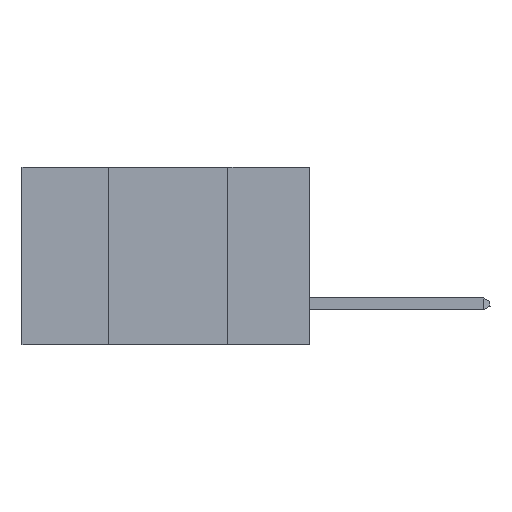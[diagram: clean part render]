
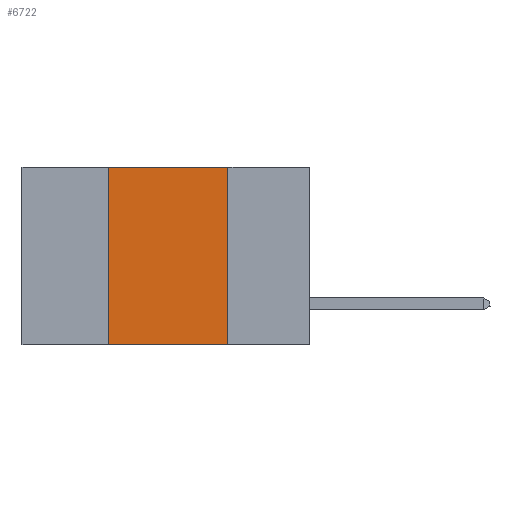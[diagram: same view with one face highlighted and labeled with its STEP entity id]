
A CAD part, left-side view. The second image highlights one B-rep face of the part: STEP entity #6722.
In plain terms, the highlighted planar face has unit normal (-1, 0, 0).
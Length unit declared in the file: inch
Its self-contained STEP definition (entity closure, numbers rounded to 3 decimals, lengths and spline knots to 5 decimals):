
#813 = LINE ( 'NONE', #24968, #1257 ) ;
#1054 = EDGE_CURVE ( 'NONE', #26137, #22305, #813, .T. ) ;
#1257 = VECTOR ( 'NONE', #18812, 39.37008 ) ;
#2636 = VERTEX_POINT ( 'NONE', #23611 ) ;
#5283 = LINE ( 'NONE', #9073, #12096 ) ;
#5435 = ORIENTED_EDGE ( 'NONE', *, *, #1054, .F. ) ;
#6722 = ADVANCED_FACE ( 'NONE', ( #33055 ), #16231, .F. ) ;
#7300 = CARTESIAN_POINT ( 'NONE',  ( 0., 0.6, 0. ) ) ;
#7421 = LINE ( 'NONE', #27315, #16544 ) ;
#9073 = CARTESIAN_POINT ( 'NONE',  ( 0., 0.42, 0. ) ) ;
#9664 = LINE ( 'NONE', #26863, #32115 ) ;
#11010 = EDGE_CURVE ( 'NONE', #23746, #26137, #7421, .T. ) ;
#12092 = EDGE_CURVE ( 'NONE', #2636, #22305, #9664, .T. ) ;
#12096 = VECTOR ( 'NONE', #26700, 39.37008 ) ;
#12722 = EDGE_LOOP ( 'NONE', ( #5435, #26218, #24633, #35678 ) ) ;
#13685 = DIRECTION ( 'NONE',  ( 0., 0., -1. ) ) ;
#14954 = DIRECTION ( 'NONE',  ( 0., -1., 0. ) ) ;
#15015 = AXIS2_PLACEMENT_3D ( 'NONE', #7300, #28284, #13685 ) ;
#16045 = DIRECTION ( 'NONE',  ( 0., -1., 0. ) ) ;
#16231 = PLANE ( 'NONE',  #15015 ) ;
#16544 = VECTOR ( 'NONE', #16045, 39.37008 ) ;
#18674 = CARTESIAN_POINT ( 'NONE',  ( 0., 0.17, -0.37 ) ) ;
#18812 = DIRECTION ( 'NONE',  ( 0., 0., -1. ) ) ;
#20277 = CARTESIAN_POINT ( 'NONE',  ( 0., 0.17, 0. ) ) ;
#21749 = CARTESIAN_POINT ( 'NONE',  ( 0., 0.42, 0. ) ) ;
#22305 = VERTEX_POINT ( 'NONE', #18674 ) ;
#23611 = CARTESIAN_POINT ( 'NONE',  ( 0., 0.42, -0.37 ) ) ;
#23746 = VERTEX_POINT ( 'NONE', #21749 ) ;
#24633 = ORIENTED_EDGE ( 'NONE', *, *, #24878, .F. ) ;
#24878 = EDGE_CURVE ( 'NONE', #2636, #23746, #5283, .T. ) ;
#24968 = CARTESIAN_POINT ( 'NONE',  ( 0., 0.17, 0. ) ) ;
#26137 = VERTEX_POINT ( 'NONE', #20277 ) ;
#26218 = ORIENTED_EDGE ( 'NONE', *, *, #11010, .F. ) ;
#26700 = DIRECTION ( 'NONE',  ( 0., 0., 1. ) ) ;
#26863 = CARTESIAN_POINT ( 'NONE',  ( 0., 0.6, -0.37 ) ) ;
#27315 = CARTESIAN_POINT ( 'NONE',  ( 0., 0.6, 0. ) ) ;
#28284 = DIRECTION ( 'NONE',  ( 1., 0., 0. ) ) ;
#32115 = VECTOR ( 'NONE', #14954, 39.37008 ) ;
#33055 = FACE_OUTER_BOUND ( 'NONE', #12722, .T. ) ;
#35678 = ORIENTED_EDGE ( 'NONE', *, *, #12092, .T. ) ;
